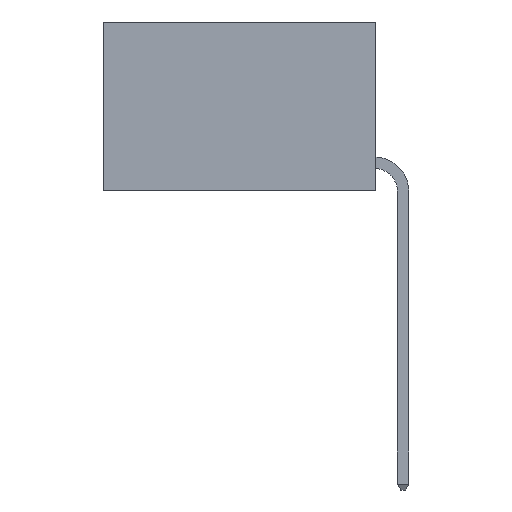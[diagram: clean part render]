
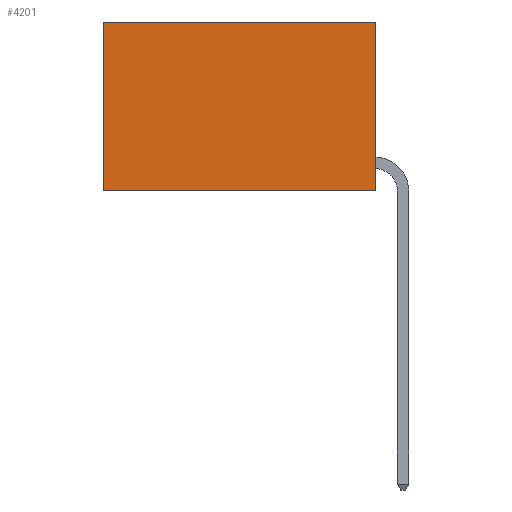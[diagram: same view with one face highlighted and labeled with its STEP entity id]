
A CAD part, left-side view. The second image highlights one B-rep face of the part: STEP entity #4201.
In plain terms, the highlighted planar face has unit normal (-1, 0, 0).
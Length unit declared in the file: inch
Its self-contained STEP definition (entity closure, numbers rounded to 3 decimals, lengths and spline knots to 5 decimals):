
#90 = LINE ( 'NONE', #735, #9232 ) ;
#735 = CARTESIAN_POINT ( 'NONE',  ( 0.2625, 0.6, 0. ) ) ;
#883 = VECTOR ( 'NONE', #2731, 39.37008 ) ;
#1590 = EDGE_CURVE ( 'NONE', #4745, #3868, #9503, .T. ) ;
#1851 = CARTESIAN_POINT ( 'NONE',  ( 0.2625, 0., 0. ) ) ;
#2731 = DIRECTION ( 'NONE',  ( 0., 1., 0. ) ) ;
#2904 = LINE ( 'NONE', #5755, #883 ) ;
#2917 = ORIENTED_EDGE ( 'NONE', *, *, #1590, .T. ) ;
#2960 = EDGE_CURVE ( 'NONE', #3868, #3334, #90, .T. ) ;
#3194 = FACE_OUTER_BOUND ( 'NONE', #6293, .T. ) ;
#3334 = VERTEX_POINT ( 'NONE', #7158 ) ;
#3568 = DIRECTION ( 'NONE',  ( 0., 1., 0. ) ) ;
#3575 = VECTOR ( 'NONE', #6231, 39.37008 ) ;
#3868 = VERTEX_POINT ( 'NONE', #8671 ) ;
#3896 = EDGE_CURVE ( 'NONE', #4745, #4911, #7627, .T. ) ;
#4201 = ADVANCED_FACE ( 'NONE', ( #3194 ), #7469, .F. ) ;
#4632 = CARTESIAN_POINT ( 'NONE',  ( 0.2625, 0., 0. ) ) ;
#4745 = VERTEX_POINT ( 'NONE', #1851 ) ;
#4911 = VERTEX_POINT ( 'NONE', #5094 ) ;
#5094 = CARTESIAN_POINT ( 'NONE',  ( 0.2625, 0., -0.37 ) ) ;
#5755 = CARTESIAN_POINT ( 'NONE',  ( 0.2625, 0., -0.37 ) ) ;
#6067 = ORIENTED_EDGE ( 'NONE', *, *, #2960, .T. ) ;
#6231 = DIRECTION ( 'NONE',  ( 0., 0., -1. ) ) ;
#6243 = CARTESIAN_POINT ( 'NONE',  ( 0.2625, 0., 0. ) ) ;
#6293 = EDGE_LOOP ( 'NONE', ( #6067, #6396, #9215, #2917 ) ) ;
#6396 = ORIENTED_EDGE ( 'NONE', *, *, #7229, .F. ) ;
#6511 = DIRECTION ( 'NONE',  ( 0., 0., -1. ) ) ;
#7158 = CARTESIAN_POINT ( 'NONE',  ( 0.2625, 0.6, -0.37 ) ) ;
#7229 = EDGE_CURVE ( 'NONE', #4911, #3334, #2904, .T. ) ;
#7469 = PLANE ( 'NONE',  #9564 ) ;
#7502 = VECTOR ( 'NONE', #3568, 39.37008 ) ;
#7627 = LINE ( 'NONE', #4632, #3575 ) ;
#8671 = CARTESIAN_POINT ( 'NONE',  ( 0.2625, 0.6, 0. ) ) ;
#8936 = DIRECTION ( 'NONE',  ( 0., 0., -1. ) ) ;
#8977 = CARTESIAN_POINT ( 'NONE',  ( 0.2625, 0., 0. ) ) ;
#9215 = ORIENTED_EDGE ( 'NONE', *, *, #3896, .F. ) ;
#9232 = VECTOR ( 'NONE', #8936, 39.37008 ) ;
#9503 = LINE ( 'NONE', #6243, #7502 ) ;
#9564 = AXIS2_PLACEMENT_3D ( 'NONE', #8977, #9798, #6511 ) ;
#9798 = DIRECTION ( 'NONE',  ( 1., 0., 0. ) ) ;
